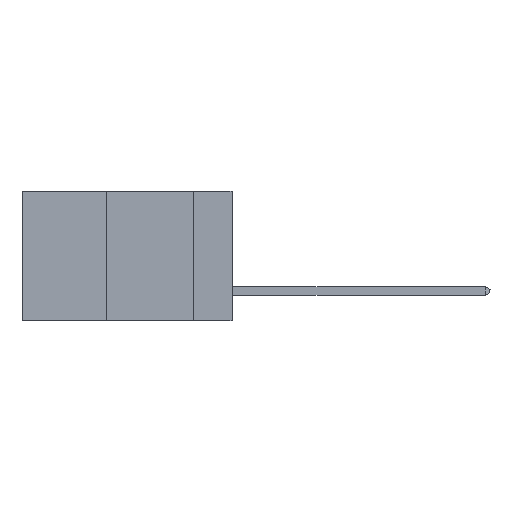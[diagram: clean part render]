
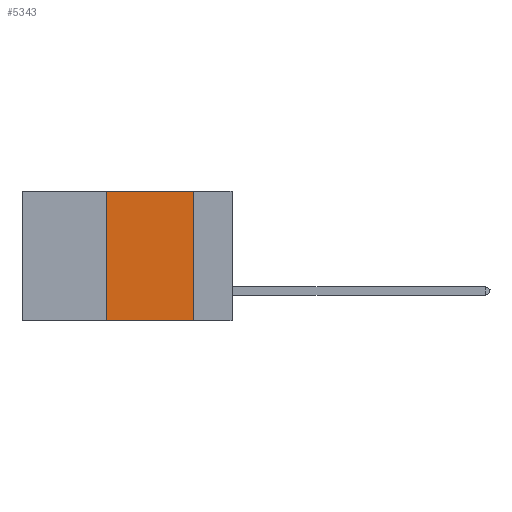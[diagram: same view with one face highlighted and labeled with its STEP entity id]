
A CAD part, left-side view. The second image highlights one B-rep face of the part: STEP entity #5343.
In plain terms, the highlighted planar face has unit normal (-1, 0, 0).
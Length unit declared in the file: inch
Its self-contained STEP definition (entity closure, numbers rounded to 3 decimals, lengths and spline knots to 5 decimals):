
#2017 = CARTESIAN_POINT ( 'NONE',  ( 0., 0.36, 0. ) ) ;
#2339 = VECTOR ( 'NONE', #32056, 39.37008 ) ;
#2983 = DIRECTION ( 'NONE',  ( 0., 0., -1. ) ) ;
#4685 = DIRECTION ( 'NONE',  ( 0., -1., 0. ) ) ;
#4866 = EDGE_CURVE ( 'NONE', #25609, #10401, #23847, .T. ) ;
#5056 = CARTESIAN_POINT ( 'NONE',  ( 0., 0.6, 0. ) ) ;
#5212 = EDGE_CURVE ( 'NONE', #10401, #34826, #12362, .T. ) ;
#5343 = ADVANCED_FACE ( 'NONE', ( #21561 ), #34651, .F. ) ;
#7401 = ORIENTED_EDGE ( 'NONE', *, *, #4866, .F. ) ;
#10401 = VERTEX_POINT ( 'NONE', #2017 ) ;
#12362 = LINE ( 'NONE', #5056, #26586 ) ;
#15048 = AXIS2_PLACEMENT_3D ( 'NONE', #22065, #28556, #2983 ) ;
#16787 = ORIENTED_EDGE ( 'NONE', *, *, #26098, .F. ) ;
#18163 = CARTESIAN_POINT ( 'NONE',  ( 0., 0.11, 0. ) ) ;
#19229 = CARTESIAN_POINT ( 'NONE',  ( 0., 0.11, -0.37 ) ) ;
#20345 = VERTEX_POINT ( 'NONE', #19229 ) ;
#21296 = ORIENTED_EDGE ( 'NONE', *, *, #5212, .F. ) ;
#21561 = FACE_OUTER_BOUND ( 'NONE', #37257, .T. ) ;
#22065 = CARTESIAN_POINT ( 'NONE',  ( 0., 0.6, 0. ) ) ;
#22083 = DIRECTION ( 'NONE',  ( 0., 0., 1. ) ) ;
#22909 = CARTESIAN_POINT ( 'NONE',  ( 0., 0.36, -0.37 ) ) ;
#23542 = LINE ( 'NONE', #31938, #2339 ) ;
#23847 = LINE ( 'NONE', #36672, #31125 ) ;
#25609 = VERTEX_POINT ( 'NONE', #22909 ) ;
#26098 = EDGE_CURVE ( 'NONE', #34826, #20345, #27611, .T. ) ;
#26586 = VECTOR ( 'NONE', #4685, 39.37008 ) ;
#27360 = CARTESIAN_POINT ( 'NONE',  ( 0., 0.11, 0. ) ) ;
#27611 = LINE ( 'NONE', #27360, #31203 ) ;
#28038 = ORIENTED_EDGE ( 'NONE', *, *, #31232, .T. ) ;
#28556 = DIRECTION ( 'NONE',  ( 1., 0., 0. ) ) ;
#31125 = VECTOR ( 'NONE', #22083, 39.37008 ) ;
#31203 = VECTOR ( 'NONE', #35944, 39.37008 ) ;
#31232 = EDGE_CURVE ( 'NONE', #25609, #20345, #23542, .T. ) ;
#31938 = CARTESIAN_POINT ( 'NONE',  ( 0., 0.6, -0.37 ) ) ;
#32056 = DIRECTION ( 'NONE',  ( 0., -1., 0. ) ) ;
#34651 = PLANE ( 'NONE',  #15048 ) ;
#34826 = VERTEX_POINT ( 'NONE', #18163 ) ;
#35944 = DIRECTION ( 'NONE',  ( 0., 0., -1. ) ) ;
#36672 = CARTESIAN_POINT ( 'NONE',  ( 0., 0.36, 0. ) ) ;
#37257 = EDGE_LOOP ( 'NONE', ( #16787, #21296, #7401, #28038 ) ) ;
